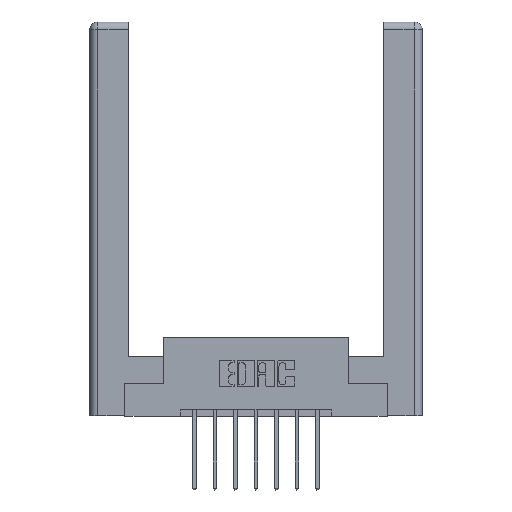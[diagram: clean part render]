
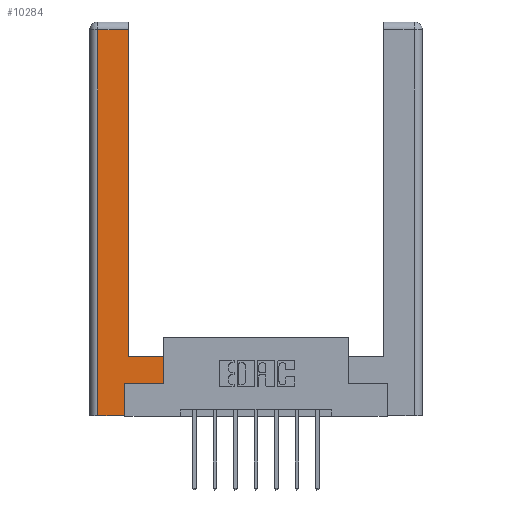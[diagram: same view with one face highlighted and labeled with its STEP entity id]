
A CAD part, top view. The second image highlights one B-rep face of the part: STEP entity #10284.
In plain terms, the highlighted planar face has unit normal (0, 0, 1).
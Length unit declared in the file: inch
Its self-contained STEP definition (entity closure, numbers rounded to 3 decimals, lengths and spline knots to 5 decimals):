
#14 = DIRECTION ( 'NONE',  ( 0., 1., 0. ) ) ;
#349 = LINE ( 'NONE', #10778, #7761 ) ;
#1134 = LINE ( 'NONE', #6909, #11184 ) ;
#1239 = VECTOR ( 'NONE', #7321, 39.37008 ) ;
#1695 = LINE ( 'NONE', #5830, #6996 ) ;
#1822 = DIRECTION ( 'NONE',  ( 1., 0., 0. ) ) ;
#1985 = EDGE_CURVE ( 'NONE', #7252, #3118, #1695, .T. ) ;
#2021 = ORIENTED_EDGE ( 'NONE', *, *, #7804, .T. ) ;
#2103 = EDGE_CURVE ( 'NONE', #3242, #8867, #6849, .T. ) ;
#2761 = EDGE_LOOP ( 'NONE', ( #5315, #5205, #12512, #6422, #2021, #3995, #4605, #8256 ) ) ;
#2812 = DIRECTION ( 'NONE',  ( 0., 1., 0. ) ) ;
#3029 = CARTESIAN_POINT ( 'NONE',  ( 0.565, 0.45, 0. ) ) ;
#3118 = VERTEX_POINT ( 'NONE', #10854 ) ;
#3145 = EDGE_CURVE ( 'NONE', #3118, #7597, #1134, .T. ) ;
#3150 = VECTOR ( 'NONE', #1822, 39.37008 ) ;
#3242 = VERTEX_POINT ( 'NONE', #5122 ) ;
#3323 = CARTESIAN_POINT ( 'NONE',  ( 0.565, 0.245, 0. ) ) ;
#3465 = CARTESIAN_POINT ( 'NONE',  ( 0.265, 0.245, 0. ) ) ;
#3706 = CARTESIAN_POINT ( 'NONE',  ( 0.0615, 0., 0. ) ) ;
#3883 = DIRECTION ( 'NONE',  ( 0., 0., -1. ) ) ;
#3937 = EDGE_CURVE ( 'NONE', #8867, #7252, #349, .T. ) ;
#3970 = DIRECTION ( 'NONE',  ( -1., 0., 0. ) ) ;
#3995 = ORIENTED_EDGE ( 'NONE', *, *, #9834, .T. ) ;
#4326 = VERTEX_POINT ( 'NONE', #12049 ) ;
#4396 = VECTOR ( 'NONE', #6453, 39.37008 ) ;
#4605 = ORIENTED_EDGE ( 'NONE', *, *, #2103, .T. ) ;
#5039 = EDGE_CURVE ( 'NONE', #7597, #4326, #5925, .T. ) ;
#5122 = CARTESIAN_POINT ( 'NONE',  ( 0.565, 0.245, 0. ) ) ;
#5205 = ORIENTED_EDGE ( 'NONE', *, *, #3145, .T. ) ;
#5315 = ORIENTED_EDGE ( 'NONE', *, *, #1985, .T. ) ;
#5399 = VERTEX_POINT ( 'NONE', #3465 ) ;
#5624 = CARTESIAN_POINT ( 'NONE',  ( 0.265, 0., 0. ) ) ;
#5643 = CARTESIAN_POINT ( 'NONE',  ( 0.265, 0.245, 0. ) ) ;
#5755 = FACE_OUTER_BOUND ( 'NONE', #2761, .T. ) ;
#5830 = CARTESIAN_POINT ( 'NONE',  ( 0.295, 3., 0. ) ) ;
#5925 = LINE ( 'NONE', #3706, #4396 ) ;
#6356 = VERTEX_POINT ( 'NONE', #7665 ) ;
#6401 = EDGE_CURVE ( 'NONE', #4326, #6356, #7538, .T. ) ;
#6422 = ORIENTED_EDGE ( 'NONE', *, *, #6401, .T. ) ;
#6453 = DIRECTION ( 'NONE',  ( 0., -1., 0. ) ) ;
#6600 = VECTOR ( 'NONE', #2812, 39.37008 ) ;
#6849 = LINE ( 'NONE', #3029, #1239 ) ;
#6909 = CARTESIAN_POINT ( 'NONE',  ( 0.0615, 2.94, 0. ) ) ;
#6973 = CARTESIAN_POINT ( 'NONE',  ( 0., 0., 0. ) ) ;
#6996 = VECTOR ( 'NONE', #14, 39.37008 ) ;
#7252 = VERTEX_POINT ( 'NONE', #11800 ) ;
#7321 = DIRECTION ( 'NONE',  ( 0., 1., 0. ) ) ;
#7538 = LINE ( 'NONE', #5624, #3150 ) ;
#7597 = VERTEX_POINT ( 'NONE', #10181 ) ;
#7665 = CARTESIAN_POINT ( 'NONE',  ( 0.265, 0., 0. ) ) ;
#7761 = VECTOR ( 'NONE', #10644, 39.37008 ) ;
#7763 = PLANE ( 'NONE',  #10509 ) ;
#7804 = EDGE_CURVE ( 'NONE', #6356, #5399, #9327, .T. ) ;
#8256 = ORIENTED_EDGE ( 'NONE', *, *, #3937, .T. ) ;
#8867 = VERTEX_POINT ( 'NONE', #10517 ) ;
#8981 = DIRECTION ( 'NONE',  ( -1., 0., 0. ) ) ;
#9250 = VECTOR ( 'NONE', #12001, 39.37008 ) ;
#9327 = LINE ( 'NONE', #5643, #6600 ) ;
#9834 = EDGE_CURVE ( 'NONE', #5399, #3242, #10650, .T. ) ;
#10181 = CARTESIAN_POINT ( 'NONE',  ( 0.0615, 2.94, 0. ) ) ;
#10284 = ADVANCED_FACE ( 'NONE', ( #5755 ), #7763, .F. ) ;
#10509 = AXIS2_PLACEMENT_3D ( 'NONE', #6973, #3883, #3970 ) ;
#10517 = CARTESIAN_POINT ( 'NONE',  ( 0.565, 0.45, 0. ) ) ;
#10644 = DIRECTION ( 'NONE',  ( -1., 0., 0. ) ) ;
#10650 = LINE ( 'NONE', #3323, #9250 ) ;
#10778 = CARTESIAN_POINT ( 'NONE',  ( 0.295, 0.45, 0. ) ) ;
#10854 = CARTESIAN_POINT ( 'NONE',  ( 0.295, 2.94, 0. ) ) ;
#11184 = VECTOR ( 'NONE', #8981, 39.37008 ) ;
#11800 = CARTESIAN_POINT ( 'NONE',  ( 0.295, 0.45, 0. ) ) ;
#12001 = DIRECTION ( 'NONE',  ( 1., 0., 0. ) ) ;
#12049 = CARTESIAN_POINT ( 'NONE',  ( 0.0615, 0., 0. ) ) ;
#12512 = ORIENTED_EDGE ( 'NONE', *, *, #5039, .T. ) ;
